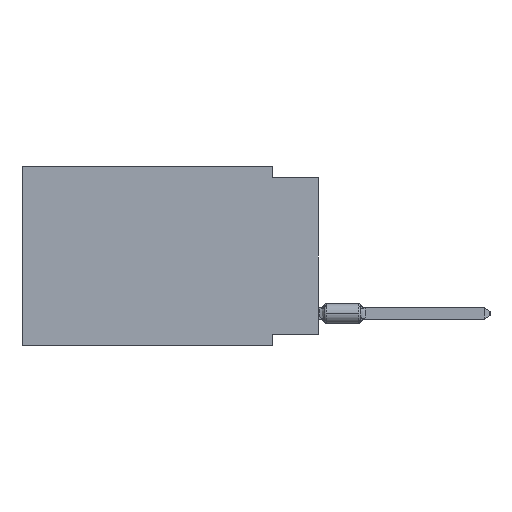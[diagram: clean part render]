
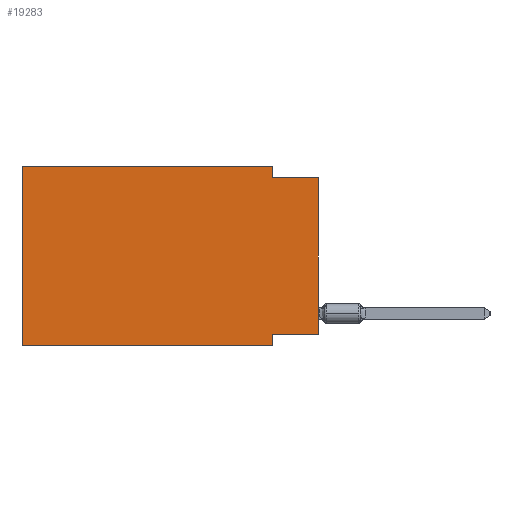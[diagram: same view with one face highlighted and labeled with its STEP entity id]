
A CAD part, left-side view. The second image highlights one B-rep face of the part: STEP entity #19283.
In plain terms, the highlighted planar face has unit normal (-1, 0, 0).
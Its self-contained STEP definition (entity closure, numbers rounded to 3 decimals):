
#142 = ORIENTED_EDGE ( 'NONE', *, *, #12874, .F. ) ;
#348 = VECTOR ( 'NONE', #21866, 1000. ) ;
#905 = EDGE_CURVE ( 'NONE', #15438, #29005, #10252, .T. ) ;
#1583 = CARTESIAN_POINT ( 'NONE',  ( 0., 0., -0.635 ) ) ;
#2330 = VERTEX_POINT ( 'NONE', #14831 ) ;
#2583 = CARTESIAN_POINT ( 'NONE',  ( 0., 16.383, 0. ) ) ;
#2764 = CARTESIAN_POINT ( 'NONE',  ( 0., 2.54, 0. ) ) ;
#2953 = EDGE_CURVE ( 'NONE', #2330, #4627, #38072, .T. ) ;
#3691 = LINE ( 'NONE', #28484, #26484 ) ;
#4176 = DIRECTION ( 'NONE',  ( 0., 0., -1. ) ) ;
#4627 = VERTEX_POINT ( 'NONE', #2583 ) ;
#5134 = DIRECTION ( 'NONE',  ( 0., 0., 1. ) ) ;
#5545 = CARTESIAN_POINT ( 'NONE',  ( 0., 0., -9.271 ) ) ;
#5648 = VERTEX_POINT ( 'NONE', #12949 ) ;
#6021 = LINE ( 'NONE', #21485, #24621 ) ;
#6198 = LINE ( 'NONE', #27940, #348 ) ;
#6335 = CARTESIAN_POINT ( 'NONE',  ( 0., 2.54, -9.906 ) ) ;
#7212 = DIRECTION ( 'NONE',  ( 1., 0., 0. ) ) ;
#8237 = VERTEX_POINT ( 'NONE', #37140 ) ;
#8265 = CARTESIAN_POINT ( 'NONE',  ( 0., 0., -0.635 ) ) ;
#8462 = LINE ( 'NONE', #8265, #9663 ) ;
#9542 = VECTOR ( 'NONE', #38672, 1000. ) ;
#9663 = VECTOR ( 'NONE', #36724, 1000. ) ;
#10252 = LINE ( 'NONE', #13490, #31815 ) ;
#10688 = VECTOR ( 'NONE', #27570, 1000. ) ;
#12874 = EDGE_CURVE ( 'NONE', #4627, #18919, #6198, .T. ) ;
#12949 = CARTESIAN_POINT ( 'NONE',  ( 0., 2.54, -9.271 ) ) ;
#13490 = CARTESIAN_POINT ( 'NONE',  ( 0., 0., 0. ) ) ;
#13523 = PLANE ( 'NONE',  #34091 ) ;
#14287 = LINE ( 'NONE', #5545, #24346 ) ;
#14609 = EDGE_LOOP ( 'NONE', ( #18698, #14965, #26594, #142, #35985, #15227, #17504, #27015 ) ) ;
#14831 = CARTESIAN_POINT ( 'NONE',  ( 0., 16.383, -9.906 ) ) ;
#14859 = CARTESIAN_POINT ( 'NONE',  ( 0., 0., -9.271 ) ) ;
#14965 = ORIENTED_EDGE ( 'NONE', *, *, #38828, .F. ) ;
#15186 = LINE ( 'NONE', #2764, #10688 ) ;
#15227 = ORIENTED_EDGE ( 'NONE', *, *, #28439, .T. ) ;
#15438 = VERTEX_POINT ( 'NONE', #14859 ) ;
#16594 = CARTESIAN_POINT ( 'NONE',  ( 0., 16.383, 0. ) ) ;
#17504 = ORIENTED_EDGE ( 'NONE', *, *, #30355, .F. ) ;
#18698 = ORIENTED_EDGE ( 'NONE', *, *, #905, .T. ) ;
#18919 = VERTEX_POINT ( 'NONE', #34370 ) ;
#18942 = VERTEX_POINT ( 'NONE', #6335 ) ;
#19283 = ADVANCED_FACE ( 'NONE', ( #34861 ), #13523, .F. ) ;
#19953 = DIRECTION ( 'NONE',  ( 0., -1., 0. ) ) ;
#21485 = CARTESIAN_POINT ( 'NONE',  ( 0., 2.54, -9.906 ) ) ;
#21866 = DIRECTION ( 'NONE',  ( 0., -1., 0. ) ) ;
#23042 = CARTESIAN_POINT ( 'NONE',  ( 0., 16.383, 0. ) ) ;
#23313 = EDGE_CURVE ( 'NONE', #18919, #8237, #15186, .T. ) ;
#24346 = VECTOR ( 'NONE', #26477, 1000. ) ;
#24387 = EDGE_CURVE ( 'NONE', #15438, #5648, #14287, .T. ) ;
#24621 = VECTOR ( 'NONE', #39778, 1000. ) ;
#26477 = DIRECTION ( 'NONE',  ( 0., 1., 0. ) ) ;
#26484 = VECTOR ( 'NONE', #19953, 1000. ) ;
#26594 = ORIENTED_EDGE ( 'NONE', *, *, #23313, .F. ) ;
#27015 = ORIENTED_EDGE ( 'NONE', *, *, #24387, .F. ) ;
#27570 = DIRECTION ( 'NONE',  ( 0., 0., -1. ) ) ;
#27940 = CARTESIAN_POINT ( 'NONE',  ( 0., 16.383, 0. ) ) ;
#28439 = EDGE_CURVE ( 'NONE', #2330, #18942, #3691, .T. ) ;
#28484 = CARTESIAN_POINT ( 'NONE',  ( 0., 16.383, -9.906 ) ) ;
#29005 = VERTEX_POINT ( 'NONE', #1583 ) ;
#30355 = EDGE_CURVE ( 'NONE', #5648, #18942, #6021, .T. ) ;
#31815 = VECTOR ( 'NONE', #5134, 1000. ) ;
#34091 = AXIS2_PLACEMENT_3D ( 'NONE', #16594, #7212, #4176 ) ;
#34370 = CARTESIAN_POINT ( 'NONE',  ( 0., 2.54, 0. ) ) ;
#34861 = FACE_OUTER_BOUND ( 'NONE', #14609, .T. ) ;
#35985 = ORIENTED_EDGE ( 'NONE', *, *, #2953, .F. ) ;
#36724 = DIRECTION ( 'NONE',  ( 0., -1., 0. ) ) ;
#37140 = CARTESIAN_POINT ( 'NONE',  ( 0., 2.54, -0.635 ) ) ;
#38072 = LINE ( 'NONE', #23042, #9542 ) ;
#38672 = DIRECTION ( 'NONE',  ( 0., 0., 1. ) ) ;
#38828 = EDGE_CURVE ( 'NONE', #8237, #29005, #8462, .T. ) ;
#39778 = DIRECTION ( 'NONE',  ( 0., 0., -1. ) ) ;
